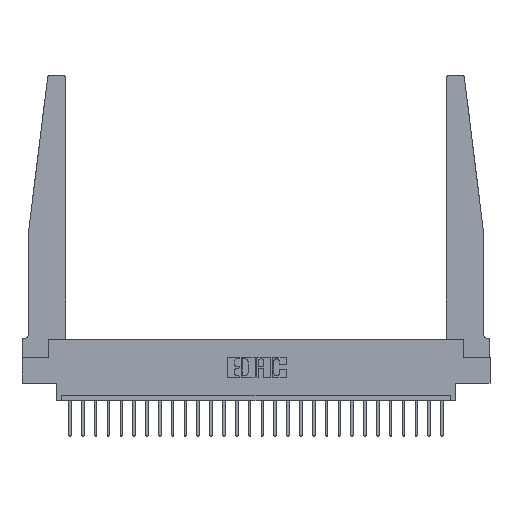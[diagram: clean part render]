
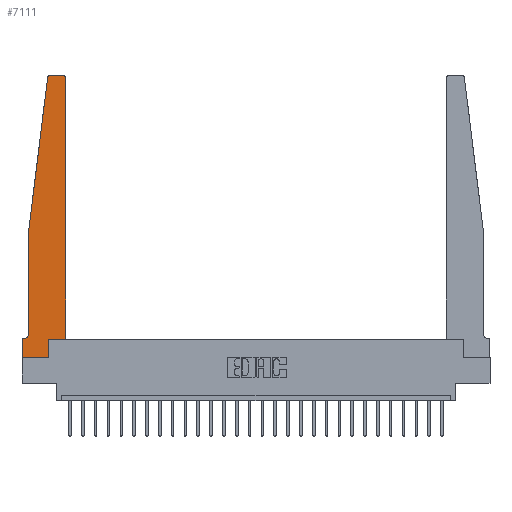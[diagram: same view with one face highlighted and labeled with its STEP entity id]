
A CAD part, top view. The second image highlights one B-rep face of the part: STEP entity #7111.
In plain terms, the highlighted planar face has unit normal (0, 0, 1).
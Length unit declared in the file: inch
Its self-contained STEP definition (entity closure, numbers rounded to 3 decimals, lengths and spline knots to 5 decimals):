
#61 = LINE ( 'NONE', #7977, #6289 ) ;
#255 = EDGE_CURVE ( 'NONE', #7884, #16647, #1086, .T. ) ;
#536 = ORIENTED_EDGE ( 'NONE', *, *, #9606, .T. ) ;
#704 = CIRCLE ( 'NONE', #10614, 0.05 ) ;
#805 = EDGE_CURVE ( 'NONE', #2518, #5490, #11251, .T. ) ;
#1086 = LINE ( 'NONE', #20883, #5760 ) ;
#2148 = VECTOR ( 'NONE', #13272, 39.37008 ) ;
#2518 = VERTEX_POINT ( 'NONE', #22673 ) ;
#2854 = LINE ( 'NONE', #10992, #4221 ) ;
#3072 = ORIENTED_EDGE ( 'NONE', *, *, #805, .T. ) ;
#3232 = ORIENTED_EDGE ( 'NONE', *, *, #15178, .T. ) ;
#3368 = CARTESIAN_POINT ( 'NONE',  ( 0., 0., 0.37 ) ) ;
#3398 = DIRECTION ( 'NONE',  ( 0., 0., 1. ) ) ;
#4041 = CARTESIAN_POINT ( 'NONE',  ( 0.27653, 2.75, 0.37 ) ) ;
#4221 = VECTOR ( 'NONE', #5304, 39.37008 ) ;
#4291 = LINE ( 'NONE', #20061, #5815 ) ;
#4391 = ORIENTED_EDGE ( 'NONE', *, *, #18985, .T. ) ;
#4578 = CARTESIAN_POINT ( 'NONE',  ( 0.015, 0.2375, 0.37 ) ) ;
#4617 = VECTOR ( 'NONE', #5961, 39.37008 ) ;
#5195 = CARTESIAN_POINT ( 'NONE',  ( 0.27653, 2.72, 0.37 ) ) ;
#5304 = DIRECTION ( 'NONE',  ( 0., 1., 0. ) ) ;
#5383 = LINE ( 'NONE', #21167, #2148 ) ;
#5438 = AXIS2_PLACEMENT_3D ( 'NONE', #5195, #19036, #12698 ) ;
#5490 = VERTEX_POINT ( 'NONE', #18661 ) ;
#5508 = EDGE_CURVE ( 'NONE', #19387, #7884, #8334, .T. ) ;
#5575 = EDGE_CURVE ( 'NONE', #18781, #21433, #8181, .T. ) ;
#5760 = VECTOR ( 'NONE', #22948, 39.37008 ) ;
#5815 = VECTOR ( 'NONE', #6229, 39.37008 ) ;
#5873 = LINE ( 'NONE', #13243, #8193 ) ;
#5961 = DIRECTION ( 'NONE',  ( 0., 1., 0. ) ) ;
#6229 = DIRECTION ( 'NONE',  ( 0., -1., 0. ) ) ;
#6275 = VERTEX_POINT ( 'NONE', #23924 ) ;
#6289 = VECTOR ( 'NONE', #15859, 39.37008 ) ;
#6300 = VERTEX_POINT ( 'NONE', #14235 ) ;
#6545 = VECTOR ( 'NONE', #23141, 39.37008 ) ;
#7111 = ADVANCED_FACE ( 'NONE', ( #20852 ), #16850, .T. ) ;
#7192 = DIRECTION ( 'NONE',  ( 1., 0., 0. ) ) ;
#7550 = ORIENTED_EDGE ( 'NONE', *, *, #13409, .T. ) ;
#7641 = CARTESIAN_POINT ( 'NONE',  ( 0.2605, 0.18, 0.37 ) ) ;
#7884 = VERTEX_POINT ( 'NONE', #10709 ) ;
#7977 = CARTESIAN_POINT ( 'NONE',  ( 0., 0., 0.37 ) ) ;
#8181 = LINE ( 'NONE', #18006, #16986 ) ;
#8193 = VECTOR ( 'NONE', #21140, 39.37008 ) ;
#8334 = CIRCLE ( 'NONE', #5438, 0.03 ) ;
#8582 = DIRECTION ( 'NONE',  ( 0., 0., -1. ) ) ;
#9279 = CARTESIAN_POINT ( 'NONE',  ( 0.065, 0.2375, 0.37 ) ) ;
#9606 = EDGE_CURVE ( 'NONE', #16471, #6275, #22424, .T. ) ;
#9709 = EDGE_CURVE ( 'NONE', #19521, #2518, #5383, .T. ) ;
#10245 = CARTESIAN_POINT ( 'NONE',  ( 0.2605, 0.18, 0.37 ) ) ;
#10614 = AXIS2_PLACEMENT_3D ( 'NONE', #4578, #8582, #16610 ) ;
#10709 = CARTESIAN_POINT ( 'NONE',  ( 0.24675, 2.72367, 0.37 ) ) ;
#10992 = CARTESIAN_POINT ( 'NONE',  ( 0.425, 0.18, 0.37 ) ) ;
#11251 = LINE ( 'NONE', #3368, #6545 ) ;
#12698 = DIRECTION ( 'NONE',  ( 1., 0., 0. ) ) ;
#12893 = CARTESIAN_POINT ( 'NONE',  ( 0.395, 2.72, 0.37 ) ) ;
#13042 = ORIENTED_EDGE ( 'NONE', *, *, #9709, .T. ) ;
#13182 = ORIENTED_EDGE ( 'NONE', *, *, #16087, .T. ) ;
#13243 = CARTESIAN_POINT ( 'NONE',  ( 0.25, 2.75, 0.37 ) ) ;
#13272 = DIRECTION ( 'NONE',  ( -1., 0., 0. ) ) ;
#13409 = EDGE_CURVE ( 'NONE', #16647, #25529, #4291, .T. ) ;
#13684 = ORIENTED_EDGE ( 'NONE', *, *, #5508, .T. ) ;
#13802 = ORIENTED_EDGE ( 'NONE', *, *, #255, .T. ) ;
#14167 = AXIS2_PLACEMENT_3D ( 'NONE', #21111, #3398, #18791 ) ;
#14235 = CARTESIAN_POINT ( 'NONE',  ( 0.2605, 0., 0.37 ) ) ;
#14584 = AXIS2_PLACEMENT_3D ( 'NONE', #12893, #18835, #7192 ) ;
#14711 = ORIENTED_EDGE ( 'NONE', *, *, #16534, .T. ) ;
#15178 = EDGE_CURVE ( 'NONE', #5490, #6300, #61, .T. ) ;
#15722 = EDGE_LOOP ( 'NONE', ( #22798, #13684, #13802, #7550, #4391, #13042, #3072, #3232, #13182, #22743, #14711, #536 ) ) ;
#15859 = DIRECTION ( 'NONE',  ( 1., 0., 0. ) ) ;
#16087 = EDGE_CURVE ( 'NONE', #6300, #18781, #23420, .T. ) ;
#16325 = CARTESIAN_POINT ( 'NONE',  ( 0.015, 0.1875, 0.37 ) ) ;
#16471 = VERTEX_POINT ( 'NONE', #24454 ) ;
#16534 = EDGE_CURVE ( 'NONE', #21433, #16471, #2854, .T. ) ;
#16610 = DIRECTION ( 'NONE',  ( -1., 0., 0. ) ) ;
#16647 = VERTEX_POINT ( 'NONE', #17573 ) ;
#16850 = PLANE ( 'NONE',  #14167 ) ;
#16986 = VECTOR ( 'NONE', #21759, 39.37008 ) ;
#17573 = CARTESIAN_POINT ( 'NONE',  ( 0.065, 1.25, 0.37 ) ) ;
#17686 = CARTESIAN_POINT ( 'NONE',  ( 0.425, 0.18, 0.37 ) ) ;
#18006 = CARTESIAN_POINT ( 'NONE',  ( 0.425, 0.18, 0.37 ) ) ;
#18661 = CARTESIAN_POINT ( 'NONE',  ( 0., 0., 0.37 ) ) ;
#18781 = VERTEX_POINT ( 'NONE', #10245 ) ;
#18791 = DIRECTION ( 'NONE',  ( 1., 0., 0. ) ) ;
#18835 = DIRECTION ( 'NONE',  ( 0., 0., 1. ) ) ;
#18985 = EDGE_CURVE ( 'NONE', #25529, #19521, #704, .T. ) ;
#19036 = DIRECTION ( 'NONE',  ( 0., 0., 1. ) ) ;
#19387 = VERTEX_POINT ( 'NONE', #4041 ) ;
#19521 = VERTEX_POINT ( 'NONE', #16325 ) ;
#20061 = CARTESIAN_POINT ( 'NONE',  ( 0.065, 1.25, 0.37 ) ) ;
#20852 = FACE_OUTER_BOUND ( 'NONE', #15722, .T. ) ;
#20883 = CARTESIAN_POINT ( 'NONE',  ( 0.065, 1.25, 0.37 ) ) ;
#20971 = EDGE_CURVE ( 'NONE', #6275, #19387, #5873, .T. ) ;
#21111 = CARTESIAN_POINT ( 'NONE',  ( 0., 0.1875, 0.37 ) ) ;
#21140 = DIRECTION ( 'NONE',  ( -1., 0., 0. ) ) ;
#21167 = CARTESIAN_POINT ( 'NONE',  ( 0.065, 0.1875, 0.37 ) ) ;
#21433 = VERTEX_POINT ( 'NONE', #17686 ) ;
#21759 = DIRECTION ( 'NONE',  ( 1., 0., 0. ) ) ;
#22424 = CIRCLE ( 'NONE', #14584, 0.03 ) ;
#22673 = CARTESIAN_POINT ( 'NONE',  ( 0., 0.1875, 0.37 ) ) ;
#22743 = ORIENTED_EDGE ( 'NONE', *, *, #5575, .T. ) ;
#22798 = ORIENTED_EDGE ( 'NONE', *, *, #20971, .T. ) ;
#22948 = DIRECTION ( 'NONE',  ( -0.122, -0.992, 0. ) ) ;
#23141 = DIRECTION ( 'NONE',  ( 0., -1., 0. ) ) ;
#23420 = LINE ( 'NONE', #7641, #4617 ) ;
#23924 = CARTESIAN_POINT ( 'NONE',  ( 0.395, 2.75, 0.37 ) ) ;
#24454 = CARTESIAN_POINT ( 'NONE',  ( 0.425, 2.72, 0.37 ) ) ;
#25529 = VERTEX_POINT ( 'NONE', #9279 ) ;
